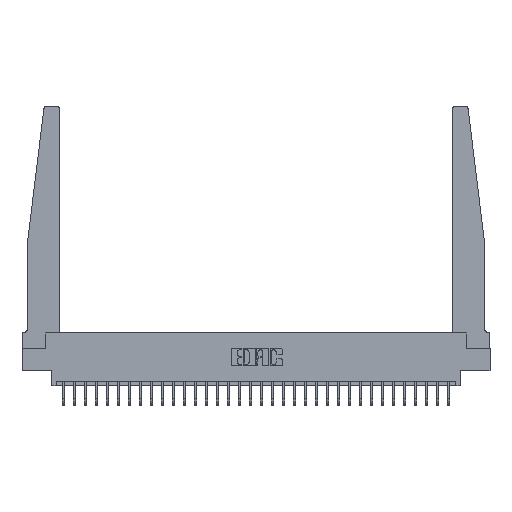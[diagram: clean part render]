
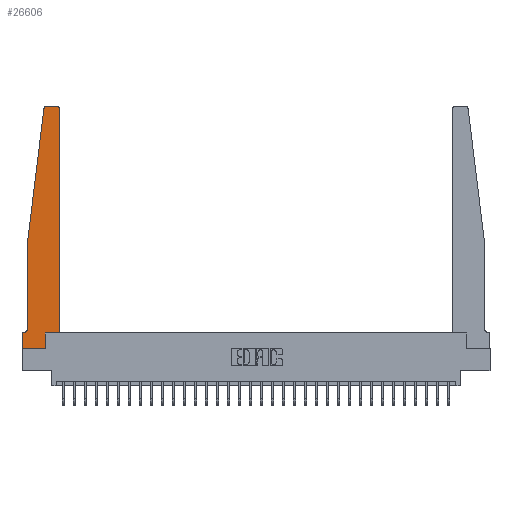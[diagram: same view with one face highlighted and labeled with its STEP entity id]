
A CAD part, top view. The second image highlights one B-rep face of the part: STEP entity #26606.
In plain terms, the highlighted planar face has unit normal (0, 0, 1).
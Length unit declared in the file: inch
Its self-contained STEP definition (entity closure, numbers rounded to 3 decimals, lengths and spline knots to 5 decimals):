
#532 = VERTEX_POINT ( 'NONE', #7016 ) ;
#631 = LINE ( 'NONE', #18362, #14493 ) ;
#1431 = DIRECTION ( 'NONE',  ( 1., 0., 0. ) ) ;
#1601 = CARTESIAN_POINT ( 'NONE',  ( 0., 0., 0.37 ) ) ;
#1862 = DIRECTION ( 'NONE',  ( 1., 0., 0. ) ) ;
#2010 = CARTESIAN_POINT ( 'NONE',  ( 0., 0., 0.37 ) ) ;
#2236 = EDGE_CURVE ( 'NONE', #2641, #21847, #18806, .T. ) ;
#2641 = VERTEX_POINT ( 'NONE', #9510 ) ;
#2742 = VERTEX_POINT ( 'NONE', #21801 ) ;
#3002 = ORIENTED_EDGE ( 'NONE', *, *, #12252, .T. ) ;
#3252 = VERTEX_POINT ( 'NONE', #5410 ) ;
#3349 = CARTESIAN_POINT ( 'NONE',  ( 0.425, 0.18, 0.37 ) ) ;
#3777 = DIRECTION ( 'NONE',  ( 0., -1., 0. ) ) ;
#4057 = ORIENTED_EDGE ( 'NONE', *, *, #2236, .T. ) ;
#5041 = CIRCLE ( 'NONE', #28306, 0.03 ) ;
#5059 = VERTEX_POINT ( 'NONE', #2010 ) ;
#5062 = EDGE_LOOP ( 'NONE', ( #12681, #18876, #25217, #6151, #29685, #24086, #3002, #30570, #4057, #11053, #28048, #29912 ) ) ;
#5410 = CARTESIAN_POINT ( 'NONE',  ( 0.395, 2.75, 0.37 ) ) ;
#5467 = LINE ( 'NONE', #15690, #30586 ) ;
#6151 = ORIENTED_EDGE ( 'NONE', *, *, #30970, .T. ) ;
#6312 = EDGE_CURVE ( 'NONE', #5059, #2641, #23137, .T. ) ;
#6688 = CARTESIAN_POINT ( 'NONE',  ( 0.2605, 0.18, 0.37 ) ) ;
#7004 = LINE ( 'NONE', #22935, #14093 ) ;
#7016 = CARTESIAN_POINT ( 'NONE',  ( 0.27653, 2.75, 0.37 ) ) ;
#7106 = VECTOR ( 'NONE', #19486, 39.37008 ) ;
#7895 = EDGE_CURVE ( 'NONE', #23201, #3252, #13035, .T. ) ;
#8088 = EDGE_CURVE ( 'NONE', #21847, #14951, #21273, .T. ) ;
#8523 = VECTOR ( 'NONE', #25421, 39.37008 ) ;
#8618 = CIRCLE ( 'NONE', #26593, 0.05 ) ;
#8673 = LINE ( 'NONE', #1601, #12421 ) ;
#8768 = CARTESIAN_POINT ( 'NONE',  ( 0.395, 2.72, 0.37 ) ) ;
#8790 = DIRECTION ( 'NONE',  ( -0.122, -0.992, 0. ) ) ;
#8988 = CARTESIAN_POINT ( 'NONE',  ( 0., 0., 0.37 ) ) ;
#9145 = DIRECTION ( 'NONE',  ( 0., -1., 0. ) ) ;
#9324 = DIRECTION ( 'NONE',  ( 0., 0., 1. ) ) ;
#9510 = CARTESIAN_POINT ( 'NONE',  ( 0.2605, 0., 0.37 ) ) ;
#9819 = CARTESIAN_POINT ( 'NONE',  ( 0.015, 0.1875, 0.37 ) ) ;
#9844 = CARTESIAN_POINT ( 'NONE',  ( 0.425, 0.18, 0.37 ) ) ;
#9884 = CARTESIAN_POINT ( 'NONE',  ( 0.2605, 0.18, 0.37 ) ) ;
#10183 = DIRECTION ( 'NONE',  ( 0., 0., 1. ) ) ;
#10342 = CARTESIAN_POINT ( 'NONE',  ( 0.425, 2.72, 0.37 ) ) ;
#10771 = FACE_OUTER_BOUND ( 'NONE', #5062, .T. ) ;
#11053 = ORIENTED_EDGE ( 'NONE', *, *, #8088, .T. ) ;
#12252 = EDGE_CURVE ( 'NONE', #16112, #5059, #8673, .T. ) ;
#12421 = VECTOR ( 'NONE', #9145, 39.37008 ) ;
#12681 = ORIENTED_EDGE ( 'NONE', *, *, #30362, .T. ) ;
#13035 = CIRCLE ( 'NONE', #27105, 0.03 ) ;
#13099 = EDGE_CURVE ( 'NONE', #2742, #24263, #8618, .T. ) ;
#14043 = LINE ( 'NONE', #30199, #18925 ) ;
#14093 = VECTOR ( 'NONE', #8790, 39.37008 ) ;
#14109 = CARTESIAN_POINT ( 'NONE',  ( 0., 0.1875, 0.37 ) ) ;
#14493 = VECTOR ( 'NONE', #18981, 39.37008 ) ;
#14740 = EDGE_CURVE ( 'NONE', #14951, #23201, #26611, .T. ) ;
#14951 = VERTEX_POINT ( 'NONE', #3349 ) ;
#15552 = DIRECTION ( 'NONE',  ( 1., 0., 0. ) ) ;
#15690 = CARTESIAN_POINT ( 'NONE',  ( 0.065, 1.25, 0.37 ) ) ;
#16112 = VERTEX_POINT ( 'NONE', #19062 ) ;
#16932 = EDGE_CURVE ( 'NONE', #24263, #16112, #14043, .T. ) ;
#18362 = CARTESIAN_POINT ( 'NONE',  ( 0.25, 2.75, 0.37 ) ) ;
#18735 = PLANE ( 'NONE',  #27981 ) ;
#18806 = LINE ( 'NONE', #6688, #29326 ) ;
#18876 = ORIENTED_EDGE ( 'NONE', *, *, #21185, .T. ) ;
#18882 = VERTEX_POINT ( 'NONE', #22387 ) ;
#18925 = VECTOR ( 'NONE', #30304, 39.37008 ) ;
#18981 = DIRECTION ( 'NONE',  ( -1., 0., 0. ) ) ;
#19062 = CARTESIAN_POINT ( 'NONE',  ( 0., 0.1875, 0.37 ) ) ;
#19486 = DIRECTION ( 'NONE',  ( 0., 1., 0. ) ) ;
#21185 = EDGE_CURVE ( 'NONE', #532, #24752, #5041, .T. ) ;
#21240 = VECTOR ( 'NONE', #15552, 39.37008 ) ;
#21273 = LINE ( 'NONE', #25728, #8523 ) ;
#21801 = CARTESIAN_POINT ( 'NONE',  ( 0.065, 0.2375, 0.37 ) ) ;
#21847 = VERTEX_POINT ( 'NONE', #9884 ) ;
#22387 = CARTESIAN_POINT ( 'NONE',  ( 0.065, 1.25, 0.37 ) ) ;
#22477 = DIRECTION ( 'NONE',  ( -1., 0., 0. ) ) ;
#22684 = CARTESIAN_POINT ( 'NONE',  ( 0.015, 0.2375, 0.37 ) ) ;
#22935 = CARTESIAN_POINT ( 'NONE',  ( 0.065, 1.25, 0.37 ) ) ;
#23137 = LINE ( 'NONE', #8988, #21240 ) ;
#23201 = VERTEX_POINT ( 'NONE', #10342 ) ;
#23292 = CARTESIAN_POINT ( 'NONE',  ( 0.24675, 2.72367, 0.37 ) ) ;
#24086 = ORIENTED_EDGE ( 'NONE', *, *, #16932, .T. ) ;
#24263 = VERTEX_POINT ( 'NONE', #9819 ) ;
#24752 = VERTEX_POINT ( 'NONE', #23292 ) ;
#25217 = ORIENTED_EDGE ( 'NONE', *, *, #26495, .T. ) ;
#25421 = DIRECTION ( 'NONE',  ( 1., 0., 0. ) ) ;
#25728 = CARTESIAN_POINT ( 'NONE',  ( 0.425, 0.18, 0.37 ) ) ;
#26495 = EDGE_CURVE ( 'NONE', #24752, #18882, #7004, .T. ) ;
#26593 = AXIS2_PLACEMENT_3D ( 'NONE', #22684, #27141, #22477 ) ;
#26606 = ADVANCED_FACE ( 'NONE', ( #10771 ), #18735, .T. ) ;
#26611 = LINE ( 'NONE', #9844, #7106 ) ;
#27105 = AXIS2_PLACEMENT_3D ( 'NONE', #8768, #30356, #1431 ) ;
#27141 = DIRECTION ( 'NONE',  ( 0., 0., -1. ) ) ;
#27197 = CARTESIAN_POINT ( 'NONE',  ( 0.27653, 2.72, 0.37 ) ) ;
#27305 = DIRECTION ( 'NONE',  ( 1., 0., 0. ) ) ;
#27981 = AXIS2_PLACEMENT_3D ( 'NONE', #14109, #9324, #1862 ) ;
#28048 = ORIENTED_EDGE ( 'NONE', *, *, #14740, .T. ) ;
#28306 = AXIS2_PLACEMENT_3D ( 'NONE', #27197, #10183, #27305 ) ;
#29326 = VECTOR ( 'NONE', #30156, 39.37008 ) ;
#29685 = ORIENTED_EDGE ( 'NONE', *, *, #13099, .T. ) ;
#29912 = ORIENTED_EDGE ( 'NONE', *, *, #7895, .T. ) ;
#30156 = DIRECTION ( 'NONE',  ( 0., 1., 0. ) ) ;
#30199 = CARTESIAN_POINT ( 'NONE',  ( 0.065, 0.1875, 0.37 ) ) ;
#30304 = DIRECTION ( 'NONE',  ( -1., 0., 0. ) ) ;
#30356 = DIRECTION ( 'NONE',  ( 0., 0., 1. ) ) ;
#30362 = EDGE_CURVE ( 'NONE', #3252, #532, #631, .T. ) ;
#30570 = ORIENTED_EDGE ( 'NONE', *, *, #6312, .T. ) ;
#30586 = VECTOR ( 'NONE', #3777, 39.37008 ) ;
#30970 = EDGE_CURVE ( 'NONE', #18882, #2742, #5467, .T. ) ;
